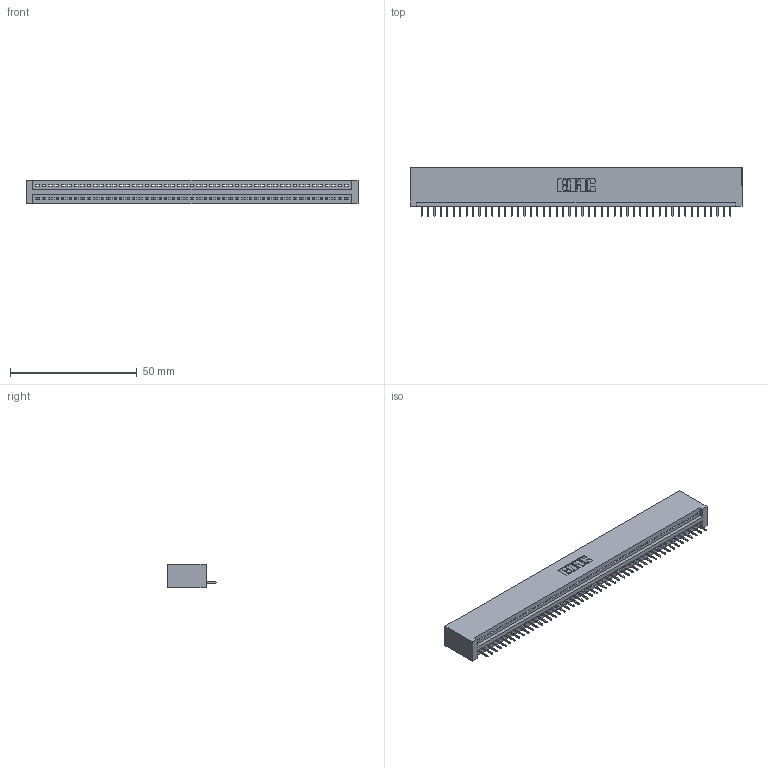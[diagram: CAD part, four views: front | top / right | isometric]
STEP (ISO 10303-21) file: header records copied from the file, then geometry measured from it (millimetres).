
FILE_DESCRIPTION (( 'STEP AP203' ), '1' );
FILE_NAME ('345-049-524-101.STEP', '2019-10-09T08:08:04', ( '' ), ( '' ), 'SwSTEP 2.0', 'SolidWorks 2016', '' );
FILE_SCHEMA (( 'CONFIG_CONTROL_DESIGN' ));
Length unit declared in the file: inch
Products named in the file (3): 345-049-524-101; 345-292-001_345-293-124; 345 Part_No Mounting Lugs
Assembly tree (50 placements, depth 2):
  345-049-524-101
    345 Part_No Mounting Lugs
    345-292-001_345-293-124  x49
Bounding box: 131.06 x 19.35 x 9.4 mm (x, y, z)
Volume: 12896.7 mm3; surface area: 16805 mm2
Topology: 50 solids, 50 shells, 3156 faces, 9137 edges, 5894 vertices
Faces by surface type: plane 2330, cylinder 826
Entity records: 35733 total; most frequent: CARTESIAN_POINT 6195, ORIENTED_EDGE 6178, DIRECTION 5395, EDGE_CURVE 3089, VECTOR 2773, LINE 2773, VERTEX_POINT 2054, AXIS2_PLACEMENT_3D 1311
